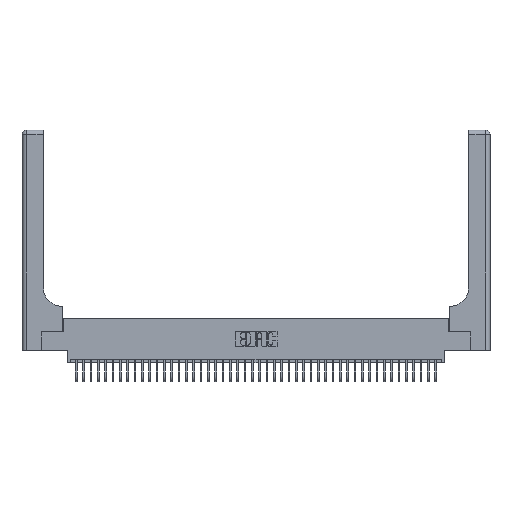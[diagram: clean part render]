
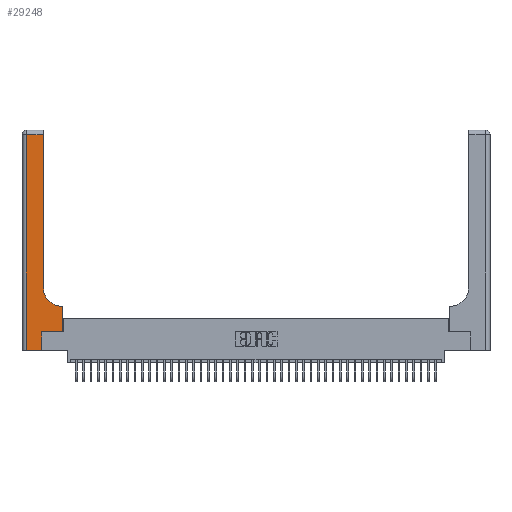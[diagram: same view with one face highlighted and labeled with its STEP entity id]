
A CAD part, top view. The second image highlights one B-rep face of the part: STEP entity #29248.
In plain terms, the highlighted planar face has unit normal (0, 0, 1).
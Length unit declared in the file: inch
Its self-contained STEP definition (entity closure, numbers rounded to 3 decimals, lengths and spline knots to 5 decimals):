
#241 = LINE ( 'NONE', #29443, #17612 ) ;
#489 = ORIENTED_EDGE ( 'NONE', *, *, #5657, .T. ) ;
#2733 = ORIENTED_EDGE ( 'NONE', *, *, #40850, .T. ) ;
#4381 = ORIENTED_EDGE ( 'NONE', *, *, #23422, .T. ) ;
#5597 = LINE ( 'NONE', #12034, #24168 ) ;
#5657 = EDGE_CURVE ( 'NONE', #14016, #9627, #5597, .T. ) ;
#5905 = EDGE_CURVE ( 'NONE', #14063, #23591, #14263, .T. ) ;
#5921 = CARTESIAN_POINT ( 'NONE',  ( 0.269, 0., 0.37 ) ) ;
#6131 = CARTESIAN_POINT ( 'NONE',  ( 0.5585, 0.25, 0.37 ) ) ;
#6797 = ORIENTED_EDGE ( 'NONE', *, *, #5905, .T. ) ;
#7038 = LINE ( 'NONE', #40141, #37066 ) ;
#7452 = CARTESIAN_POINT ( 'NONE',  ( 0., 3., 0.37 ) ) ;
#7665 = CARTESIAN_POINT ( 'NONE',  ( 0.5585, 0.25, 0.37 ) ) ;
#8146 = CARTESIAN_POINT ( 'NONE',  ( 0.269, 0.25, 0.37 ) ) ;
#8790 = VERTEX_POINT ( 'NONE', #20945 ) ;
#9627 = VERTEX_POINT ( 'NONE', #5921 ) ;
#9883 = CARTESIAN_POINT ( 'NONE',  ( 0.2915, 3., 0.37 ) ) ;
#10093 = DIRECTION ( 'NONE',  ( 0., 1., 0. ) ) ;
#10761 = AXIS2_PLACEMENT_3D ( 'NONE', #39107, #18168, #42614 ) ;
#10953 = DIRECTION ( 'NONE',  ( -1., 0., 0. ) ) ;
#12034 = CARTESIAN_POINT ( 'NONE',  ( 0., 0., 0.37 ) ) ;
#14016 = VERTEX_POINT ( 'NONE', #31852 ) ;
#14063 = VERTEX_POINT ( 'NONE', #7665 ) ;
#14263 = LINE ( 'NONE', #6131, #22487 ) ;
#14287 = CARTESIAN_POINT ( 'NONE',  ( 0.5415, 0.6, 0.37 ) ) ;
#14839 = EDGE_CURVE ( 'NONE', #30748, #14063, #41187, .T. ) ;
#15371 = CARTESIAN_POINT ( 'NONE',  ( 0.269, 0.25, 0.37 ) ) ;
#16340 = VECTOR ( 'NONE', #24336, 39.37008 ) ;
#17612 = VECTOR ( 'NONE', #22505, 39.37008 ) ;
#18168 = DIRECTION ( 'NONE',  ( 0., 0., -1. ) ) ;
#19188 = DIRECTION ( 'NONE',  ( -1., 0., 0. ) ) ;
#19901 = AXIS2_PLACEMENT_3D ( 'NONE', #7452, #31930, #10953 ) ;
#20043 = VERTEX_POINT ( 'NONE', #31574 ) ;
#20945 = CARTESIAN_POINT ( 'NONE',  ( 0.2915, 0.85, 0.37 ) ) ;
#21489 = VECTOR ( 'NONE', #43342, 39.37008 ) ;
#22107 = ORIENTED_EDGE ( 'NONE', *, *, #25289, .T. ) ;
#22451 = DIRECTION ( 'NONE',  ( 1., 0., 0. ) ) ;
#22487 = VECTOR ( 'NONE', #34211, 39.37008 ) ;
#22505 = DIRECTION ( 'NONE',  ( -1., 0., 0. ) ) ;
#23422 = EDGE_CURVE ( 'NONE', #35182, #20043, #7038, .T. ) ;
#23591 = VERTEX_POINT ( 'NONE', #27064 ) ;
#24088 = EDGE_LOOP ( 'NONE', ( #36825, #4381, #26868, #489, #2733, #25572, #6797, #36484, #22107 ) ) ;
#24168 = VECTOR ( 'NONE', #22451, 39.37008 ) ;
#24336 = DIRECTION ( 'NONE',  ( 0., -1., 0. ) ) ;
#25289 = EDGE_CURVE ( 'NONE', #31938, #8790, #37821, .T. ) ;
#25572 = ORIENTED_EDGE ( 'NONE', *, *, #14839, .T. ) ;
#25713 = LINE ( 'NONE', #41722, #16340 ) ;
#26868 = ORIENTED_EDGE ( 'NONE', *, *, #26981, .T. ) ;
#26981 = EDGE_CURVE ( 'NONE', #20043, #14016, #25713, .T. ) ;
#27064 = CARTESIAN_POINT ( 'NONE',  ( 0.5585, 0.6, 0.37 ) ) ;
#27713 = FACE_OUTER_BOUND ( 'NONE', #24088, .T. ) ;
#28447 = PLANE ( 'NONE',  #19901 ) ;
#29248 = ADVANCED_FACE ( 'NONE', ( #27713 ), #28447, .F. ) ;
#29443 = CARTESIAN_POINT ( 'NONE',  ( 0.2915, 0.6, 0.37 ) ) ;
#30748 = VERTEX_POINT ( 'NONE', #8146 ) ;
#31070 = CARTESIAN_POINT ( 'NONE',  ( 0.269, 0., 0.37 ) ) ;
#31364 = CARTESIAN_POINT ( 'NONE',  ( 0.2915, 2.94, 0.37 ) ) ;
#31574 = CARTESIAN_POINT ( 'NONE',  ( 0.06, 2.94, 0.37 ) ) ;
#31760 = EDGE_CURVE ( 'NONE', #8790, #35182, #36301, .T. ) ;
#31852 = CARTESIAN_POINT ( 'NONE',  ( 0.06, 0., 0.37 ) ) ;
#31930 = DIRECTION ( 'NONE',  ( 0., 0., -1. ) ) ;
#31938 = VERTEX_POINT ( 'NONE', #14287 ) ;
#32616 = VECTOR ( 'NONE', #10093, 39.37008 ) ;
#32699 = EDGE_CURVE ( 'NONE', #23591, #31938, #241, .T. ) ;
#34211 = DIRECTION ( 'NONE',  ( 0., 1., 0. ) ) ;
#34346 = DIRECTION ( 'NONE',  ( 0., 1., 0. ) ) ;
#35182 = VERTEX_POINT ( 'NONE', #31364 ) ;
#36301 = LINE ( 'NONE', #9883, #44495 ) ;
#36484 = ORIENTED_EDGE ( 'NONE', *, *, #32699, .T. ) ;
#36825 = ORIENTED_EDGE ( 'NONE', *, *, #31760, .T. ) ;
#37066 = VECTOR ( 'NONE', #19188, 39.37008 ) ;
#37821 = CIRCLE ( 'NONE', #10761, 0.25 ) ;
#39107 = CARTESIAN_POINT ( 'NONE',  ( 0.5415, 0.85, 0.37 ) ) ;
#40141 = CARTESIAN_POINT ( 'NONE',  ( 0., 2.94, 0.37 ) ) ;
#40850 = EDGE_CURVE ( 'NONE', #9627, #30748, #44044, .T. ) ;
#41187 = LINE ( 'NONE', #15371, #21489 ) ;
#41722 = CARTESIAN_POINT ( 'NONE',  ( 0.06, 3., 0.37 ) ) ;
#42614 = DIRECTION ( 'NONE',  ( 1., 0., 0. ) ) ;
#43342 = DIRECTION ( 'NONE',  ( 1., 0., 0. ) ) ;
#44044 = LINE ( 'NONE', #31070, #32616 ) ;
#44495 = VECTOR ( 'NONE', #34346, 39.37008 ) ;
